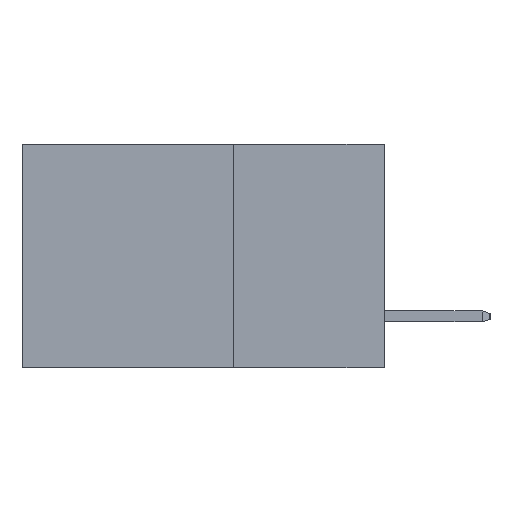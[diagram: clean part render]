
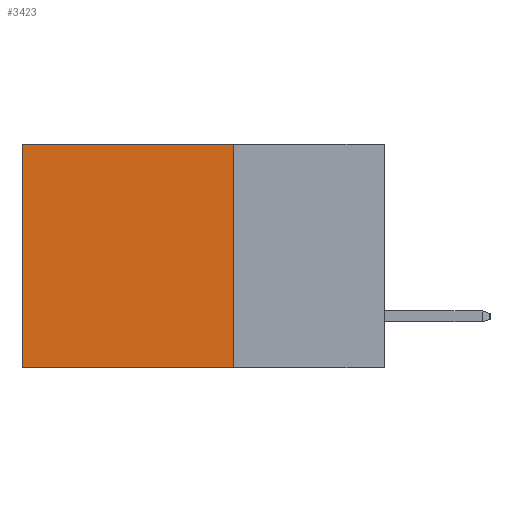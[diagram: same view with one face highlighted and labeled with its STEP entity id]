
A CAD part, left-side view. The second image highlights one B-rep face of the part: STEP entity #3423.
In plain terms, the highlighted planar face has unit normal (-1, 0, 0).
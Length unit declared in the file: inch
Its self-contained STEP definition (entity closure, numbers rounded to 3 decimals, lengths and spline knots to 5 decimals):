
#240 = CARTESIAN_POINT ( 'NONE',  ( 0.298, 0.6, 0. ) ) ;
#272 = DIRECTION ( 'NONE',  ( 0., 0., -1. ) ) ;
#452 = LINE ( 'NONE', #1098, #6093 ) ;
#1098 = CARTESIAN_POINT ( 'NONE',  ( 0.298, 0.25, 0. ) ) ;
#1472 = VERTEX_POINT ( 'NONE', #3146 ) ;
#2555 = LINE ( 'NONE', #7302, #10615 ) ;
#3146 = CARTESIAN_POINT ( 'NONE',  ( 0.298, 0.25, -0.37 ) ) ;
#3423 = ADVANCED_FACE ( 'NONE', ( #5321 ), #9994, .F. ) ;
#3873 = CARTESIAN_POINT ( 'NONE',  ( 0.298, 0.6, -0.37 ) ) ;
#4192 = EDGE_LOOP ( 'NONE', ( #4966, #10541, #11761, #6580 ) ) ;
#4966 = ORIENTED_EDGE ( 'NONE', *, *, #5816, .T. ) ;
#5079 = LINE ( 'NONE', #240, #13249 ) ;
#5276 = AXIS2_PLACEMENT_3D ( 'NONE', #5469, #8469, #272 ) ;
#5321 = FACE_OUTER_BOUND ( 'NONE', #4192, .T. ) ;
#5469 = CARTESIAN_POINT ( 'NONE',  ( 0.298, 0.25, 0. ) ) ;
#5816 = EDGE_CURVE ( 'NONE', #13890, #12574, #5079, .T. ) ;
#6093 = VECTOR ( 'NONE', #7803, 39.37008 ) ;
#6580 = ORIENTED_EDGE ( 'NONE', *, *, #13165, .T. ) ;
#7012 = DIRECTION ( 'NONE',  ( 0., 0., -1. ) ) ;
#7109 = LINE ( 'NONE', #13092, #10318 ) ;
#7302 = CARTESIAN_POINT ( 'NONE',  ( 0.298, 0.25, -0.37 ) ) ;
#7788 = EDGE_CURVE ( 'NONE', #1472, #12574, #2555, .T. ) ;
#7803 = DIRECTION ( 'NONE',  ( 0., 0., -1. ) ) ;
#8469 = DIRECTION ( 'NONE',  ( 1., 0., 0. ) ) ;
#9994 = PLANE ( 'NONE',  #5276 ) ;
#10042 = DIRECTION ( 'NONE',  ( 0., 1., 0. ) ) ;
#10318 = VECTOR ( 'NONE', #10042, 39.37008 ) ;
#10541 = ORIENTED_EDGE ( 'NONE', *, *, #7788, .F. ) ;
#10548 = EDGE_CURVE ( 'NONE', #12884, #1472, #452, .T. ) ;
#10615 = VECTOR ( 'NONE', #12590, 39.37008 ) ;
#11761 = ORIENTED_EDGE ( 'NONE', *, *, #10548, .F. ) ;
#11946 = CARTESIAN_POINT ( 'NONE',  ( 0.298, 0.25, 0. ) ) ;
#12467 = CARTESIAN_POINT ( 'NONE',  ( 0.298, 0.6, 0. ) ) ;
#12574 = VERTEX_POINT ( 'NONE', #3873 ) ;
#12590 = DIRECTION ( 'NONE',  ( 0., 1., 0. ) ) ;
#12884 = VERTEX_POINT ( 'NONE', #11946 ) ;
#13092 = CARTESIAN_POINT ( 'NONE',  ( 0.298, 0.25, 0. ) ) ;
#13165 = EDGE_CURVE ( 'NONE', #12884, #13890, #7109, .T. ) ;
#13249 = VECTOR ( 'NONE', #7012, 39.37008 ) ;
#13890 = VERTEX_POINT ( 'NONE', #12467 ) ;
